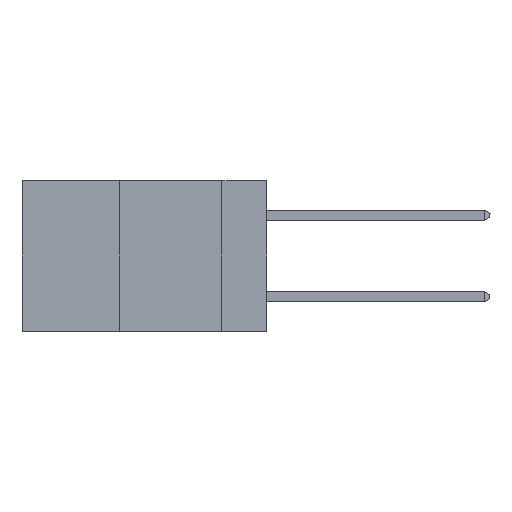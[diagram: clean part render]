
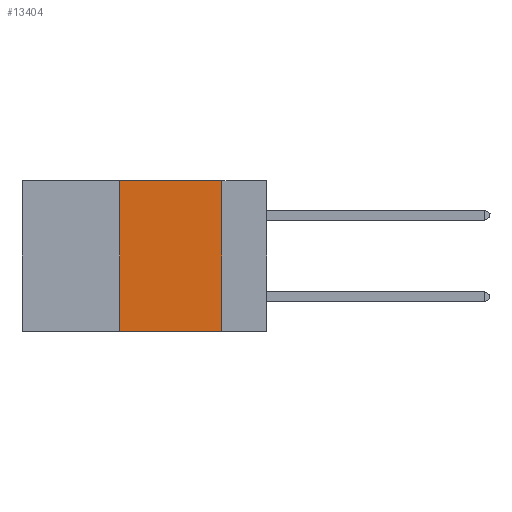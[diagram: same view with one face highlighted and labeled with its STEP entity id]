
A CAD part, left-side view. The second image highlights one B-rep face of the part: STEP entity #13404.
In plain terms, the highlighted planar face has unit normal (-1, 0, 0).
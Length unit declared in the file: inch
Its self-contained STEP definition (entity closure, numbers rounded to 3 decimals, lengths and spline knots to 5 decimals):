
#1685 = LINE ( 'NONE', #12209, #15743 ) ;
#2249 = PLANE ( 'NONE',  #4585 ) ;
#2383 = DIRECTION ( 'NONE',  ( 0., 0., -1. ) ) ;
#3024 = EDGE_CURVE ( 'NONE', #13225, #5368, #12506, .T. ) ;
#4585 = AXIS2_PLACEMENT_3D ( 'NONE', #15041, #6576, #2383 ) ;
#4694 = ORIENTED_EDGE ( 'NONE', *, *, #17771, .F. ) ;
#5368 = VERTEX_POINT ( 'NONE', #8856 ) ;
#6576 = DIRECTION ( 'NONE',  ( 1., 0., 0. ) ) ;
#6807 = CARTESIAN_POINT ( 'NONE',  ( 0., 0.36, 0. ) ) ;
#6984 = DIRECTION ( 'NONE',  ( 0., -1., 0. ) ) ;
#7015 = ORIENTED_EDGE ( 'NONE', *, *, #9147, .T. ) ;
#7495 = LINE ( 'NONE', #6807, #10978 ) ;
#8002 = EDGE_CURVE ( 'NONE', #8697, #13225, #7495, .T. ) ;
#8498 = CARTESIAN_POINT ( 'NONE',  ( 0., 0.36, -0.37 ) ) ;
#8697 = VERTEX_POINT ( 'NONE', #8498 ) ;
#8856 = CARTESIAN_POINT ( 'NONE',  ( 0., 0.11, 0. ) ) ;
#9147 = EDGE_CURVE ( 'NONE', #8697, #15619, #15094, .T. ) ;
#9901 = VECTOR ( 'NONE', #6984, 39.37008 ) ;
#10148 = CARTESIAN_POINT ( 'NONE',  ( 0., 0.6, -0.37 ) ) ;
#10978 = VECTOR ( 'NONE', #16889, 39.37008 ) ;
#11289 = CARTESIAN_POINT ( 'NONE',  ( 0., 0.11, -0.37 ) ) ;
#11333 = CARTESIAN_POINT ( 'NONE',  ( 0., 0.6, 0. ) ) ;
#11630 = ORIENTED_EDGE ( 'NONE', *, *, #3024, .F. ) ;
#12028 = DIRECTION ( 'NONE',  ( 0., 0., -1. ) ) ;
#12209 = CARTESIAN_POINT ( 'NONE',  ( 0., 0.11, 0. ) ) ;
#12506 = LINE ( 'NONE', #11333, #9901 ) ;
#12778 = ORIENTED_EDGE ( 'NONE', *, *, #8002, .F. ) ;
#13225 = VERTEX_POINT ( 'NONE', #15018 ) ;
#13404 = ADVANCED_FACE ( 'NONE', ( #15254 ), #2249, .F. ) ;
#13781 = VECTOR ( 'NONE', #14488, 39.37008 ) ;
#14488 = DIRECTION ( 'NONE',  ( 0., -1., 0. ) ) ;
#15018 = CARTESIAN_POINT ( 'NONE',  ( 0., 0.36, 0. ) ) ;
#15041 = CARTESIAN_POINT ( 'NONE',  ( 0., 0.6, 0. ) ) ;
#15094 = LINE ( 'NONE', #10148, #13781 ) ;
#15254 = FACE_OUTER_BOUND ( 'NONE', #17190, .T. ) ;
#15619 = VERTEX_POINT ( 'NONE', #11289 ) ;
#15743 = VECTOR ( 'NONE', #12028, 39.37008 ) ;
#16889 = DIRECTION ( 'NONE',  ( 0., 0., 1. ) ) ;
#17190 = EDGE_LOOP ( 'NONE', ( #4694, #11630, #12778, #7015 ) ) ;
#17771 = EDGE_CURVE ( 'NONE', #5368, #15619, #1685, .T. ) ;
